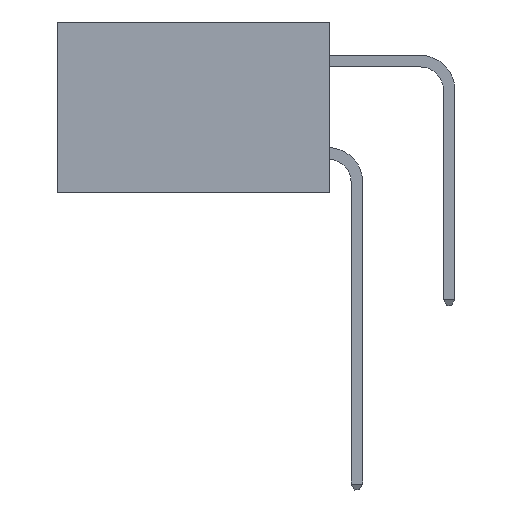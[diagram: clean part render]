
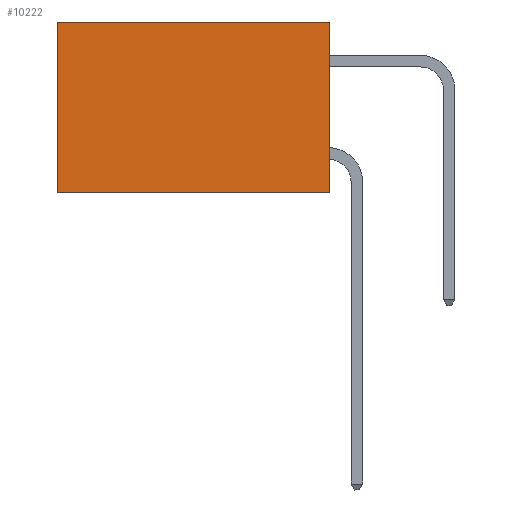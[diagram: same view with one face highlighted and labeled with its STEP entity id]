
A CAD part, left-side view. The second image highlights one B-rep face of the part: STEP entity #10222.
In plain terms, the highlighted planar face has unit normal (-1, 0, 0).
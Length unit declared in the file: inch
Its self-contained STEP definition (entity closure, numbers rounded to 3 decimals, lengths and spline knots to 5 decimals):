
#82 = CARTESIAN_POINT ( 'NONE',  ( 0.277, 0.59, -0.37 ) ) ;
#228 = LINE ( 'NONE', #2402, #6813 ) ;
#275 = DIRECTION ( 'NONE',  ( 0., 0., -1. ) ) ;
#395 = DIRECTION ( 'NONE',  ( 0., 0., -1. ) ) ;
#790 = CARTESIAN_POINT ( 'NONE',  ( 0.277, 0., 0. ) ) ;
#974 = ORIENTED_EDGE ( 'NONE', *, *, #5211, .T. ) ;
#1225 = DIRECTION ( 'NONE',  ( 0., 1., 0. ) ) ;
#1263 = LINE ( 'NONE', #9147, #5577 ) ;
#1960 = CARTESIAN_POINT ( 'NONE',  ( 0.277, 0.59, 0. ) ) ;
#2130 = EDGE_CURVE ( 'NONE', #4152, #3310, #4624, .T. ) ;
#2360 = VECTOR ( 'NONE', #1225, 39.37008 ) ;
#2402 = CARTESIAN_POINT ( 'NONE',  ( 0.277, 0.59, -0.37 ) ) ;
#2579 = DIRECTION ( 'NONE',  ( 0., 0., -1. ) ) ;
#3002 = ORIENTED_EDGE ( 'NONE', *, *, #3896, .T. ) ;
#3310 = VERTEX_POINT ( 'NONE', #82 ) ;
#3779 = PLANE ( 'NONE',  #4430 ) ;
#3896 = EDGE_CURVE ( 'NONE', #6888, #3310, #228, .T. ) ;
#4152 = VERTEX_POINT ( 'NONE', #7371 ) ;
#4385 = LINE ( 'NONE', #10410, #8683 ) ;
#4430 = AXIS2_PLACEMENT_3D ( 'NONE', #10535, #5548, #395 ) ;
#4624 = LINE ( 'NONE', #8306, #2360 ) ;
#5211 = EDGE_CURVE ( 'NONE', #9877, #6888, #1263, .T. ) ;
#5273 = ORIENTED_EDGE ( 'NONE', *, *, #2130, .F. ) ;
#5548 = DIRECTION ( 'NONE',  ( 1., 0., 0. ) ) ;
#5577 = VECTOR ( 'NONE', #8633, 39.37008 ) ;
#6813 = VECTOR ( 'NONE', #2579, 39.37008 ) ;
#6888 = VERTEX_POINT ( 'NONE', #1960 ) ;
#7371 = CARTESIAN_POINT ( 'NONE',  ( 0.277, 0., -0.37 ) ) ;
#7585 = ORIENTED_EDGE ( 'NONE', *, *, #10806, .F. ) ;
#8306 = CARTESIAN_POINT ( 'NONE',  ( 0.277, 0., -0.37 ) ) ;
#8633 = DIRECTION ( 'NONE',  ( 0., 1., 0. ) ) ;
#8683 = VECTOR ( 'NONE', #275, 39.37008 ) ;
#9147 = CARTESIAN_POINT ( 'NONE',  ( 0.277, 0., 0. ) ) ;
#9877 = VERTEX_POINT ( 'NONE', #790 ) ;
#10216 = FACE_OUTER_BOUND ( 'NONE', #10647, .T. ) ;
#10222 = ADVANCED_FACE ( 'NONE', ( #10216 ), #3779, .F. ) ;
#10410 = CARTESIAN_POINT ( 'NONE',  ( 0.277, 0., -0.37 ) ) ;
#10535 = CARTESIAN_POINT ( 'NONE',  ( 0.277, 0., -0.37 ) ) ;
#10647 = EDGE_LOOP ( 'NONE', ( #3002, #5273, #7585, #974 ) ) ;
#10806 = EDGE_CURVE ( 'NONE', #9877, #4152, #4385, .T. ) ;
